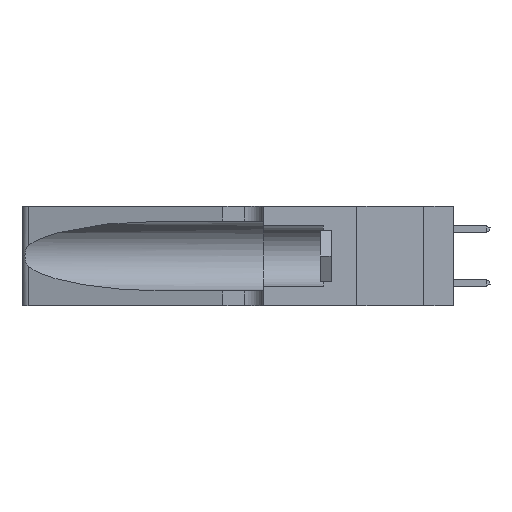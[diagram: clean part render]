
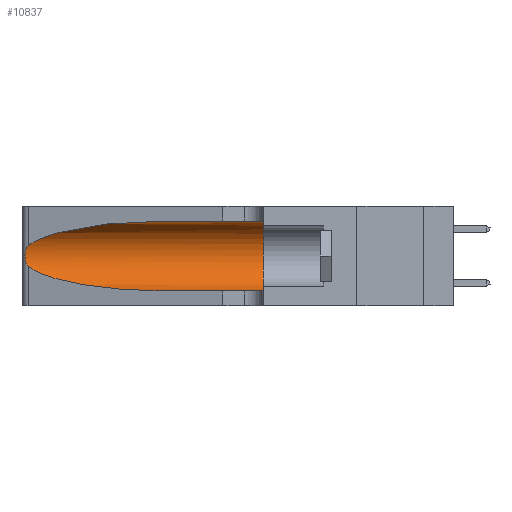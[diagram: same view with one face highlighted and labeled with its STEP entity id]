
A CAD part, left-side view. The second image highlights one B-rep face of the part: STEP entity #10837.
In plain terms, the highlighted cylindrical face has radius 3.308 mm (diameter 6.617 mm), a partial arc.
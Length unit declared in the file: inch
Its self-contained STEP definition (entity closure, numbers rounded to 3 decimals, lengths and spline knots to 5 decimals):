
#1095 = CARTESIAN_POINT ( 'NONE',  ( 0.1305, 0.72297, 0.31525 ) ) ;
#1350 = CARTESIAN_POINT ( 'NONE',  ( 0.25555, 1.22994, 0.2215 ) ) ;
#1983 = VERTEX_POINT ( 'NONE', #19706 ) ;
#2647 = DIRECTION ( 'NONE',  ( 0., -1., 0. ) ) ;
#3388 = VERTEX_POINT ( 'NONE', #24529 ) ;
#3461 = CARTESIAN_POINT ( 'NONE',  ( 0.26075, 1.23896, 0.178 ) ) ;
#3495 = CARTESIAN_POINT ( 'NONE',  ( 0.25487, 1.22718, 0.14631 ) ) ;
#3502 = CARTESIAN_POINT ( 'NONE',  ( 0.2373, 1.15595, 0.28018 ) ) ;
#3606 = CARTESIAN_POINT ( 'NONE',  ( 0.18966, 0.96281, 0.31525 ) ) ;
#4203 = CARTESIAN_POINT ( 'NONE',  ( 0.1305, 0.72297, 0.05475 ) ) ;
#4331 =( BOUNDED_CURVE ( )  B_SPLINE_CURVE ( 3, ( #1095, #3606, #3502, #26098 ),
 .UNSPECIFIED., .F., .F. ) 
 B_SPLINE_CURVE_WITH_KNOTS ( ( 4, 4 ),
 ( 1.5708, 2.84003 ),
 .UNSPECIFIED. ) 
 CURVE ( )  GEOMETRIC_REPRESENTATION_ITEM ( )  RATIONAL_B_SPLINE_CURVE ( ( 1., 0.87, 0.87, 1. ) ) 
 REPRESENTATION_ITEM ( '' )  );
#4513 = ORIENTED_EDGE ( 'NONE', *, *, #17150, .F. ) ;
#4763 = CIRCLE ( 'NONE', #17959, 0.13025 ) ;
#4856 = CARTESIAN_POINT ( 'NONE',  ( 0.1305, 0.35, 0.185 ) ) ;
#4942 = CARTESIAN_POINT ( 'NONE',  ( 0.1305, 1.61858, 0.31525 ) ) ;
#4988 = VECTOR ( 'NONE', #25734, 39.37008 ) ;
#5937 = CARTESIAN_POINT ( 'NONE',  ( 0.25856, 1.23593, 0.16098 ) ) ;
#6155 = B_SPLINE_CURVE_WITH_KNOTS ( 'NONE', 3,
 ( #28358, #1350, #10428, #14817, #17058, #28670, #21816, #3461, #17356, #5937, #12731, #28571, #19324, #12624 ),
 .UNSPECIFIED., .F., .F.,
 ( 4, 2, 2, 2, 2, 2, 4 ),
 ( 0., 0.00027, 0.00053, 0.00107, 0.0016, 0.00187, 0.00214 ),
 .UNSPECIFIED. ) ;
#6566 = DIRECTION ( 'NONE',  ( 0., 0., 1. ) ) ;
#7764 = ORIENTED_EDGE ( 'NONE', *, *, #21462, .F. ) ;
#8719 =( BOUNDED_CURVE ( )  B_SPLINE_CURVE ( 3, ( #3495, #25892, #26220, #4203 ),
 .UNSPECIFIED., .F., .F. ) 
 B_SPLINE_CURVE_WITH_KNOTS ( ( 4, 4 ),
 ( 3.44316, 4.71239 ),
 .UNSPECIFIED. ) 
 CURVE ( )  GEOMETRIC_REPRESENTATION_ITEM ( )  RATIONAL_B_SPLINE_CURVE ( ( 1., 0.87, 0.87, 1. ) ) 
 REPRESENTATION_ITEM ( '' )  );
#9018 = CARTESIAN_POINT ( 'NONE',  ( 0.25487, 1.22718, 0.14631 ) ) ;
#9333 = CARTESIAN_POINT ( 'NONE',  ( 0.1305, 1.61858, 0.185 ) ) ;
#10428 = CARTESIAN_POINT ( 'NONE',  ( 0.25639, 1.23184, 0.21858 ) ) ;
#10802 = AXIS2_PLACEMENT_3D ( 'NONE', #9333, #2647, #24973 ) ;
#10837 = ADVANCED_FACE ( 'NONE', ( #16292 ), #20878, .F. ) ;
#11495 = EDGE_CURVE ( 'NONE', #12187, #1983, #8719, .T. ) ;
#12187 = VERTEX_POINT ( 'NONE', #9018 ) ;
#12624 = CARTESIAN_POINT ( 'NONE',  ( 0.25487, 1.22718, 0.14631 ) ) ;
#12731 = CARTESIAN_POINT ( 'NONE',  ( 0.25789, 1.23486, 0.15765 ) ) ;
#14693 = LINE ( 'NONE', #4942, #24258 ) ;
#14817 = CARTESIAN_POINT ( 'NONE',  ( 0.25787, 1.23484, 0.2124 ) ) ;
#14984 = ORIENTED_EDGE ( 'NONE', *, *, #11495, .T. ) ;
#15486 = ORIENTED_EDGE ( 'NONE', *, *, #22274, .T. ) ;
#15866 = CARTESIAN_POINT ( 'NONE',  ( 0.1305, 0.35, 0.05475 ) ) ;
#16127 = DIRECTION ( 'NONE',  ( 0., 1., 0. ) ) ;
#16251 = EDGE_LOOP ( 'NONE', ( #24124, #25249, #14984, #15486, #4513, #7764 ) ) ;
#16292 = FACE_OUTER_BOUND ( 'NONE', #16251, .T. ) ;
#17000 = VERTEX_POINT ( 'NONE', #24522 ) ;
#17058 = CARTESIAN_POINT ( 'NONE',  ( 0.25854, 1.2359, 0.20912 ) ) ;
#17150 = EDGE_CURVE ( 'NONE', #3388, #22641, #4763, .T. ) ;
#17356 = CARTESIAN_POINT ( 'NONE',  ( 0.26017, 1.23833, 0.17102 ) ) ;
#17959 = AXIS2_PLACEMENT_3D ( 'NONE', #4856, #16127, #6566 ) ;
#18647 = DIRECTION ( 'NONE',  ( 0., -1., 0. ) ) ;
#19324 = CARTESIAN_POINT ( 'NONE',  ( 0.25555, 1.22993, 0.14849 ) ) ;
#19706 = CARTESIAN_POINT ( 'NONE',  ( 0.1305, 0.72297, 0.05475 ) ) ;
#20275 = EDGE_CURVE ( 'NONE', #20421, #17000, #4331, .T. ) ;
#20421 = VERTEX_POINT ( 'NONE', #27023 ) ;
#20878 = CYLINDRICAL_SURFACE ( 'NONE', #10802, 0.13025 ) ;
#21462 = EDGE_CURVE ( 'NONE', #20421, #3388, #14693, .T. ) ;
#21732 = EDGE_CURVE ( 'NONE', #17000, #12187, #6155, .T. ) ;
#21816 = CARTESIAN_POINT ( 'NONE',  ( 0.26075, 1.23896, 0.19203 ) ) ;
#22274 = EDGE_CURVE ( 'NONE', #1983, #22641, #25238, .T. ) ;
#22641 = VERTEX_POINT ( 'NONE', #15866 ) ;
#24124 = ORIENTED_EDGE ( 'NONE', *, *, #20275, .T. ) ;
#24258 = VECTOR ( 'NONE', #18647, 39.37008 ) ;
#24522 = CARTESIAN_POINT ( 'NONE',  ( 0.25487, 1.22718, 0.22369 ) ) ;
#24529 = CARTESIAN_POINT ( 'NONE',  ( 0.1305, 0.35, 0.31525 ) ) ;
#24973 = DIRECTION ( 'NONE',  ( 0., 0., -1. ) ) ;
#25238 = LINE ( 'NONE', #26017, #4988 ) ;
#25249 = ORIENTED_EDGE ( 'NONE', *, *, #21732, .T. ) ;
#25734 = DIRECTION ( 'NONE',  ( 0., -1., 0. ) ) ;
#25892 = CARTESIAN_POINT ( 'NONE',  ( 0.2373, 1.15595, 0.08982 ) ) ;
#26017 = CARTESIAN_POINT ( 'NONE',  ( 0.1305, 1.61858, 0.05475 ) ) ;
#26098 = CARTESIAN_POINT ( 'NONE',  ( 0.25487, 1.22718, 0.22369 ) ) ;
#26220 = CARTESIAN_POINT ( 'NONE',  ( 0.18966, 0.96281, 0.05475 ) ) ;
#27023 = CARTESIAN_POINT ( 'NONE',  ( 0.1305, 0.72297, 0.31525 ) ) ;
#28358 = CARTESIAN_POINT ( 'NONE',  ( 0.25487, 1.22718, 0.22369 ) ) ;
#28571 = CARTESIAN_POINT ( 'NONE',  ( 0.25639, 1.23186, 0.15144 ) ) ;
#28670 = CARTESIAN_POINT ( 'NONE',  ( 0.26018, 1.23835, 0.19895 ) ) ;
